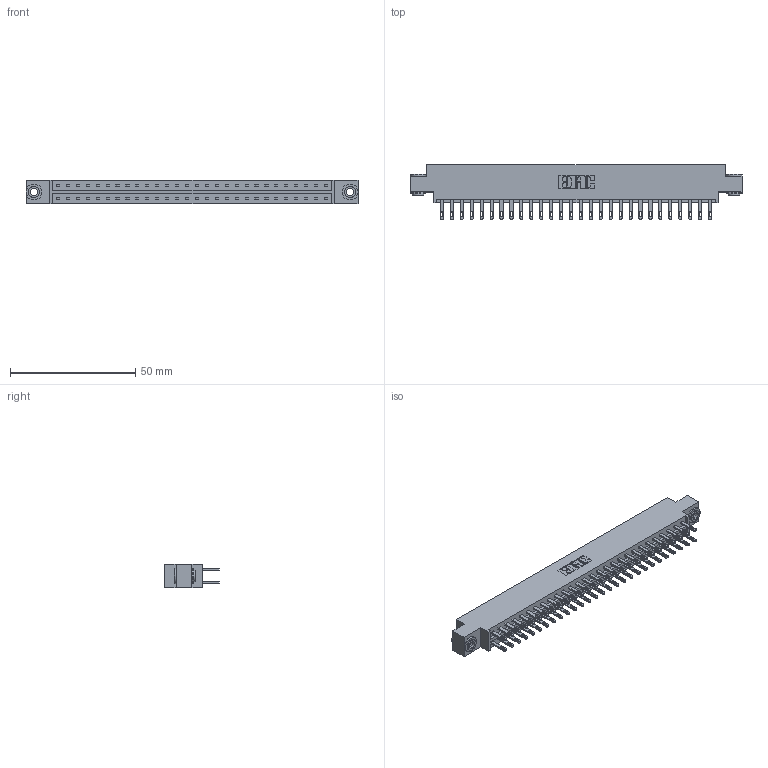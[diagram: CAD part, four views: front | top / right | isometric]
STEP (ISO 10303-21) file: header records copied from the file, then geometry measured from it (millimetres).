
FILE_DESCRIPTION (( 'STEP AP203' ), '1' );
FILE_NAME ('333-056-500-803.STEP', '2018-08-04T04:28:25', ( '' ), ( '' ), 'SwSTEP 2.0', 'SolidWorks 2016', '' );
FILE_SCHEMA (( 'CONFIG_CONTROL_DESIGN' ));
Length unit declared in the file: inch
Products named in the file (4): 345-250-002_345-250-002-102; 333-056-500-803; 333 Part_Offset - .156 Dia - TH; 345-292-001_345-293-100
Assembly tree (59 placements, depth 2):
  333-056-500-803
    333 Part_Offset - .156 Dia - TH
    345-292-001_345-293-100  x56
    345-250-002_345-250-002-102  x2
Bounding box: 132.49 x 21.85 x 9.4 mm (x, y, z)
Volume: 13357.9 mm3; surface area: 16699.9 mm2
Topology: 59 solids, 59 shells, 2844 faces, 8631 edges, 5750 vertices
Faces by surface type: plane 1764, cylinder 1072, cone 8
Entity records: 20536 total; most frequent: CARTESIAN_POINT 3397, ORIENTED_EDGE 3326, DIRECTION 2961, EDGE_CURVE 1663, LINE 1507, VECTOR 1507, VERTEX_POINT 1106, AXIS2_PLACEMENT_3D 727
